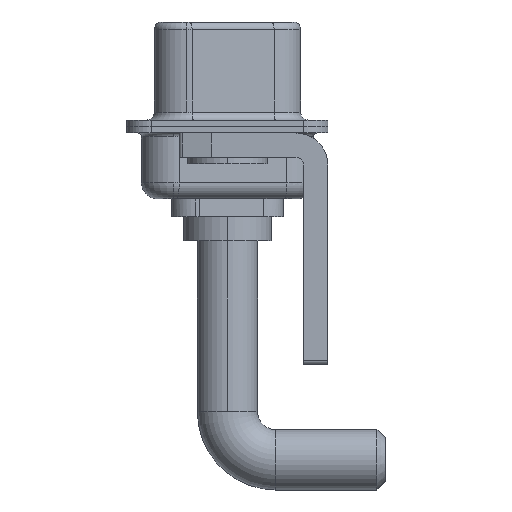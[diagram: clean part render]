
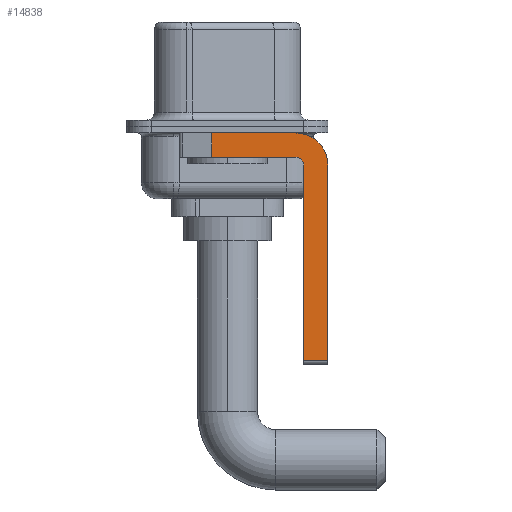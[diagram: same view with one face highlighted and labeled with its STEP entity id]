
A CAD part, left-side view. The second image highlights one B-rep face of the part: STEP entity #14838.
In plain terms, the highlighted planar face has unit normal (-1, 0, 0).
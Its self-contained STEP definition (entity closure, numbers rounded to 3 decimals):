
#29 = CARTESIAN_POINT ( 'NONE',  ( -2.9, 0.978, -1.9 ) ) ;
#352 = CARTESIAN_POINT ( 'NONE',  ( -2.9, -4.25, -2.4 ) ) ;
#496 = ORIENTED_EDGE ( 'NONE', *, *, #14229, .T. ) ;
#795 = DIRECTION ( 'NONE',  ( 0., 0., -1. ) ) ;
#836 = DIRECTION ( 'NONE',  ( 0., -1., 0. ) ) ;
#837 = EDGE_LOOP ( 'NONE', ( #7749, #496, #7103, #14146, #3944, #5219, #9694, #4136 ) ) ;
#943 = EDGE_CURVE ( 'NONE', #5233, #7016, #11654, .T. ) ;
#1352 = VERTEX_POINT ( 'NONE', #7428 ) ;
#1732 = DIRECTION ( 'NONE',  ( -1., 0., 0. ) ) ;
#1849 = VERTEX_POINT ( 'NONE', #5813 ) ;
#1895 = CARTESIAN_POINT ( 'NONE',  ( -2.9, -4.25, -2.4 ) ) ;
#2121 = LINE ( 'NONE', #16357, #6644 ) ;
#2245 = CARTESIAN_POINT ( 'NONE',  ( -2.9, -6.25, -2.4 ) ) ;
#2265 = AXIS2_PLACEMENT_3D ( 'NONE', #352, #8216, #3150 ) ;
#2481 = LINE ( 'NONE', #14318, #7834 ) ;
#3070 = FACE_OUTER_BOUND ( 'NONE', #837, .T. ) ;
#3150 = DIRECTION ( 'NONE',  ( 0., 0., -1. ) ) ;
#3197 = EDGE_CURVE ( 'NONE', #1352, #1849, #4305, .T. ) ;
#3220 = VERTEX_POINT ( 'NONE', #10752 ) ;
#3457 = CARTESIAN_POINT ( 'NONE',  ( -2.9, -4.25, -1.9 ) ) ;
#3944 = ORIENTED_EDGE ( 'NONE', *, *, #3197, .F. ) ;
#4136 = ORIENTED_EDGE ( 'NONE', *, *, #943, .F. ) ;
#4305 = LINE ( 'NONE', #14700, #14173 ) ;
#5219 = ORIENTED_EDGE ( 'NONE', *, *, #5751, .T. ) ;
#5233 = VERTEX_POINT ( 'NONE', #10384 ) ;
#5342 = DIRECTION ( 'NONE',  ( 0., 0., -1. ) ) ;
#5751 = EDGE_CURVE ( 'NONE', #1352, #7662, #2121, .T. ) ;
#5766 = VECTOR ( 'NONE', #15637, 1000. ) ;
#5813 = CARTESIAN_POINT ( 'NONE',  ( -2.9, -4.75, -2.4 ) ) ;
#6195 = CARTESIAN_POINT ( 'NONE',  ( -2.9, 0.978, -0.4 ) ) ;
#6297 = CARTESIAN_POINT ( 'NONE',  ( -2.9, 0.978, -1.9 ) ) ;
#6574 = VERTEX_POINT ( 'NONE', #6195 ) ;
#6644 = VECTOR ( 'NONE', #836, 1000. ) ;
#7016 = VERTEX_POINT ( 'NONE', #7196 ) ;
#7103 = ORIENTED_EDGE ( 'NONE', *, *, #7529, .F. ) ;
#7196 = CARTESIAN_POINT ( 'NONE',  ( -2.9, -6.25, -2.4 ) ) ;
#7428 = CARTESIAN_POINT ( 'NONE',  ( -2.9, -4.75, -14.55 ) ) ;
#7529 = EDGE_CURVE ( 'NONE', #3220, #12502, #9653, .T. ) ;
#7662 = VERTEX_POINT ( 'NONE', #9128 ) ;
#7749 = ORIENTED_EDGE ( 'NONE', *, *, #8757, .F. ) ;
#7818 = LINE ( 'NONE', #29, #5766 ) ;
#7834 = VECTOR ( 'NONE', #10453, 1000. ) ;
#8139 = CIRCLE ( 'NONE', #8669, 0.5 ) ;
#8216 = DIRECTION ( 'NONE',  ( 1., 0., 0. ) ) ;
#8669 = AXIS2_PLACEMENT_3D ( 'NONE', #1895, #1732, #9527 ) ;
#8757 = EDGE_CURVE ( 'NONE', #6574, #5233, #2481, .T. ) ;
#9128 = CARTESIAN_POINT ( 'NONE',  ( -2.9, -6.25, -14.55 ) ) ;
#9527 = DIRECTION ( 'NONE',  ( 0., 0., 1. ) ) ;
#9653 = LINE ( 'NONE', #3457, #15968 ) ;
#9694 = ORIENTED_EDGE ( 'NONE', *, *, #10105, .F. ) ;
#10105 = EDGE_CURVE ( 'NONE', #7016, #7662, #16400, .T. ) ;
#10384 = CARTESIAN_POINT ( 'NONE',  ( -2.9, -4.25, -0.4 ) ) ;
#10453 = DIRECTION ( 'NONE',  ( 0., -1., 0. ) ) ;
#10533 = EDGE_CURVE ( 'NONE', #1849, #3220, #8139, .T. ) ;
#10752 = CARTESIAN_POINT ( 'NONE',  ( -2.9, -4.25, -1.9 ) ) ;
#11563 = CARTESIAN_POINT ( 'NONE',  ( -2.9, -4.25, -2.4 ) ) ;
#11654 = CIRCLE ( 'NONE', #16293, 2. ) ;
#12502 = VERTEX_POINT ( 'NONE', #6297 ) ;
#13107 = DIRECTION ( 'NONE',  ( 1., 0., 0. ) ) ;
#14146 = ORIENTED_EDGE ( 'NONE', *, *, #10533, .F. ) ;
#14173 = VECTOR ( 'NONE', #14452, 1000. ) ;
#14229 = EDGE_CURVE ( 'NONE', #6574, #12502, #7818, .T. ) ;
#14318 = CARTESIAN_POINT ( 'NONE',  ( -2.9, 3., -0.4 ) ) ;
#14452 = DIRECTION ( 'NONE',  ( 0., 0., 1. ) ) ;
#14700 = CARTESIAN_POINT ( 'NONE',  ( -2.9, -4.75, -14.8 ) ) ;
#14820 = PLANE ( 'NONE',  #2265 ) ;
#14838 = ADVANCED_FACE ( 'NONE', ( #3070 ), #14820, .F. ) ;
#14886 = DIRECTION ( 'NONE',  ( 0., 1., 0. ) ) ;
#15637 = DIRECTION ( 'NONE',  ( 0., 0., -1. ) ) ;
#15968 = VECTOR ( 'NONE', #14886, 1000. ) ;
#16293 = AXIS2_PLACEMENT_3D ( 'NONE', #11563, #13107, #5342 ) ;
#16349 = VECTOR ( 'NONE', #795, 1000. ) ;
#16357 = CARTESIAN_POINT ( 'NONE',  ( -2.9, -4.25, -14.55 ) ) ;
#16400 = LINE ( 'NONE', #2245, #16349 ) ;
